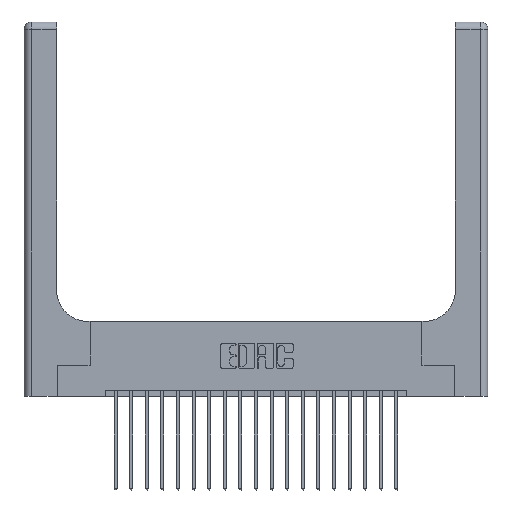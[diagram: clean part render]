
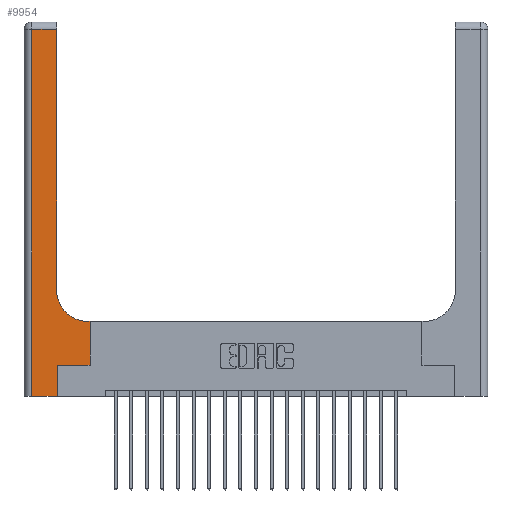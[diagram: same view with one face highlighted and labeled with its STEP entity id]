
A CAD part, top view. The second image highlights one B-rep face of the part: STEP entity #9954.
In plain terms, the highlighted planar face has unit normal (0, 0, 1).
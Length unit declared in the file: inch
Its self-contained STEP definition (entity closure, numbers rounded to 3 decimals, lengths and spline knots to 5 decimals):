
#460 = AXIS2_PLACEMENT_3D ( 'NONE', #7739, #20786, #7843 ) ;
#1253 = CARTESIAN_POINT ( 'NONE',  ( 0.26, 3., 0.37 ) ) ;
#1589 = ORIENTED_EDGE ( 'NONE', *, *, #17703, .T. ) ;
#2178 = AXIS2_PLACEMENT_3D ( 'NONE', #8605, #15148, #6997 ) ;
#2201 = LINE ( 'NONE', #15405, #3660 ) ;
#2478 = FACE_OUTER_BOUND ( 'NONE', #10318, .T. ) ;
#2603 = VERTEX_POINT ( 'NONE', #6345 ) ;
#2856 = LINE ( 'NONE', #1253, #15217 ) ;
#3018 = CARTESIAN_POINT ( 'NONE',  ( 0.06, 3., 0.37 ) ) ;
#3286 = VECTOR ( 'NONE', #14845, 39.37008 ) ;
#3497 = CARTESIAN_POINT ( 'NONE',  ( 0.265, 0., 0.37 ) ) ;
#3660 = VECTOR ( 'NONE', #8751, 39.37008 ) ;
#3775 = PLANE ( 'NONE',  #2178 ) ;
#3798 = EDGE_CURVE ( 'NONE', #2603, #17460, #2201, .T. ) ;
#4504 = CARTESIAN_POINT ( 'NONE',  ( 0.26, 2.94, 0.37 ) ) ;
#4648 = ORIENTED_EDGE ( 'NONE', *, *, #12568, .T. ) ;
#4717 = VECTOR ( 'NONE', #12067, 39.37008 ) ;
#5933 = CIRCLE ( 'NONE', #460, 0.25 ) ;
#6345 = CARTESIAN_POINT ( 'NONE',  ( 0.528, 0.25, 0.37 ) ) ;
#6503 = DIRECTION ( 'NONE',  ( 0., 1., 0. ) ) ;
#6601 = ORIENTED_EDGE ( 'NONE', *, *, #14131, .T. ) ;
#6812 = CARTESIAN_POINT ( 'NONE',  ( 0.265, 0.25, 0.37 ) ) ;
#6997 = DIRECTION ( 'NONE',  ( -1., 0., 0. ) ) ;
#7233 = CARTESIAN_POINT ( 'NONE',  ( 0., 2.94, 0.37 ) ) ;
#7351 = VERTEX_POINT ( 'NONE', #4504 ) ;
#7713 = DIRECTION ( 'NONE',  ( 1., 0., 0. ) ) ;
#7739 = CARTESIAN_POINT ( 'NONE',  ( 0.51, 0.85, 0.37 ) ) ;
#7843 = DIRECTION ( 'NONE',  ( 1., 0., 0. ) ) ;
#8325 = ORIENTED_EDGE ( 'NONE', *, *, #12146, .T. ) ;
#8520 = ORIENTED_EDGE ( 'NONE', *, *, #20045, .T. ) ;
#8533 = CARTESIAN_POINT ( 'NONE',  ( 0.06, 0., 0.37 ) ) ;
#8605 = CARTESIAN_POINT ( 'NONE',  ( 0., 3., 0.37 ) ) ;
#8751 = DIRECTION ( 'NONE',  ( 0., 1., 0. ) ) ;
#9426 = DIRECTION ( 'NONE',  ( -1., 0., 0. ) ) ;
#9508 = CARTESIAN_POINT ( 'NONE',  ( 0.51, 0.6, 0.37 ) ) ;
#9565 = DIRECTION ( 'NONE',  ( 0., -1., 0. ) ) ;
#9578 = VERTEX_POINT ( 'NONE', #11090 ) ;
#9901 = CARTESIAN_POINT ( 'NONE',  ( 0.26, 0.85, 0.37 ) ) ;
#9915 = LINE ( 'NONE', #16667, #3286 ) ;
#9954 = ADVANCED_FACE ( 'NONE', ( #2478 ), #3775, .F. ) ;
#10054 = VECTOR ( 'NONE', #9426, 39.37008 ) ;
#10318 = EDGE_LOOP ( 'NONE', ( #8325, #16440, #8520, #1589, #4648, #6601, #12871, #19283, #17160 ) ) ;
#10934 = LINE ( 'NONE', #17347, #17343 ) ;
#11090 = CARTESIAN_POINT ( 'NONE',  ( 0.265, 0., 0.37 ) ) ;
#11205 = EDGE_CURVE ( 'NONE', #12217, #16892, #5933, .T. ) ;
#11492 = CARTESIAN_POINT ( 'NONE',  ( 0.528, 0.6, 0.37 ) ) ;
#11595 = EDGE_CURVE ( 'NONE', #17460, #12217, #18843, .T. ) ;
#11642 = VECTOR ( 'NONE', #9565, 39.37008 ) ;
#12067 = DIRECTION ( 'NONE',  ( -1., 0., 0. ) ) ;
#12146 = EDGE_CURVE ( 'NONE', #16892, #7351, #2856, .T. ) ;
#12217 = VERTEX_POINT ( 'NONE', #9508 ) ;
#12277 = LINE ( 'NONE', #7233, #4717 ) ;
#12539 = CARTESIAN_POINT ( 'NONE',  ( 0.26, 0.6, 0.37 ) ) ;
#12568 = EDGE_CURVE ( 'NONE', #9578, #16586, #12941, .T. ) ;
#12871 = ORIENTED_EDGE ( 'NONE', *, *, #3798, .T. ) ;
#12941 = LINE ( 'NONE', #3497, #20674 ) ;
#14131 = EDGE_CURVE ( 'NONE', #16586, #2603, #9915, .T. ) ;
#14845 = DIRECTION ( 'NONE',  ( 1., 0., 0. ) ) ;
#15148 = DIRECTION ( 'NONE',  ( 0., 0., -1. ) ) ;
#15217 = VECTOR ( 'NONE', #20842, 39.37008 ) ;
#15334 = CARTESIAN_POINT ( 'NONE',  ( 0.06, 2.94, 0.37 ) ) ;
#15405 = CARTESIAN_POINT ( 'NONE',  ( 0.528, 0.25, 0.37 ) ) ;
#16440 = ORIENTED_EDGE ( 'NONE', *, *, #16689, .T. ) ;
#16586 = VERTEX_POINT ( 'NONE', #6812 ) ;
#16667 = CARTESIAN_POINT ( 'NONE',  ( 0.265, 0.25, 0.37 ) ) ;
#16689 = EDGE_CURVE ( 'NONE', #7351, #20805, #12277, .T. ) ;
#16892 = VERTEX_POINT ( 'NONE', #9901 ) ;
#17160 = ORIENTED_EDGE ( 'NONE', *, *, #11205, .T. ) ;
#17343 = VECTOR ( 'NONE', #7713, 39.37008 ) ;
#17347 = CARTESIAN_POINT ( 'NONE',  ( 0., 0., 0.37 ) ) ;
#17460 = VERTEX_POINT ( 'NONE', #11492 ) ;
#17692 = LINE ( 'NONE', #3018, #11642 ) ;
#17703 = EDGE_CURVE ( 'NONE', #17868, #9578, #10934, .T. ) ;
#17868 = VERTEX_POINT ( 'NONE', #8533 ) ;
#18843 = LINE ( 'NONE', #12539, #10054 ) ;
#19283 = ORIENTED_EDGE ( 'NONE', *, *, #11595, .T. ) ;
#20045 = EDGE_CURVE ( 'NONE', #20805, #17868, #17692, .T. ) ;
#20674 = VECTOR ( 'NONE', #6503, 39.37008 ) ;
#20786 = DIRECTION ( 'NONE',  ( 0., 0., -1. ) ) ;
#20805 = VERTEX_POINT ( 'NONE', #15334 ) ;
#20842 = DIRECTION ( 'NONE',  ( 0., 1., 0. ) ) ;
